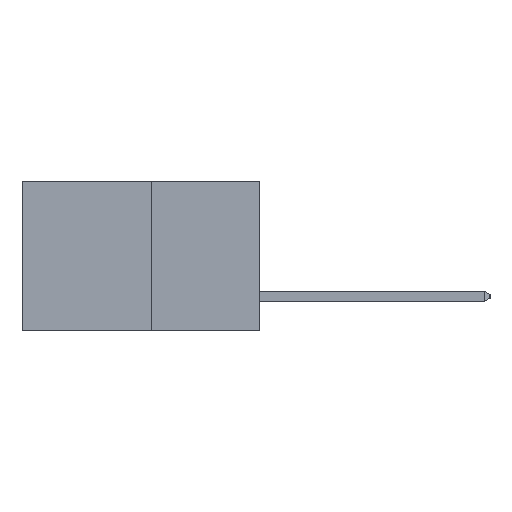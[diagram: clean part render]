
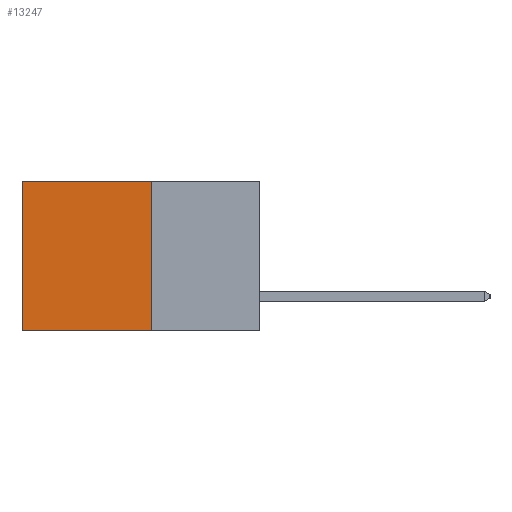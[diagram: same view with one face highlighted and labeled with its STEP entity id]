
A CAD part, left-side view. The second image highlights one B-rep face of the part: STEP entity #13247.
In plain terms, the highlighted planar face has unit normal (-1, 0, 0).
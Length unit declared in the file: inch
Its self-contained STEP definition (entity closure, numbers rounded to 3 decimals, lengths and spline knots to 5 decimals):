
#35 = VECTOR ( 'NONE', #3221, 39.37008 ) ;
#95 = CARTESIAN_POINT ( 'NONE',  ( 0.277, 0.27, -0.37 ) ) ;
#238 = ORIENTED_EDGE ( 'NONE', *, *, #1452, .F. ) ;
#782 = DIRECTION ( 'NONE',  ( 0., 1., 0. ) ) ;
#844 = CARTESIAN_POINT ( 'NONE',  ( 0.277, 0.59, -0.37 ) ) ;
#1452 = EDGE_CURVE ( 'NONE', #14737, #11930, #11901, .T. ) ;
#1801 = EDGE_CURVE ( 'NONE', #3575, #6230, #9563, .T. ) ;
#3221 = DIRECTION ( 'NONE',  ( 0., 0., -1. ) ) ;
#3575 = VERTEX_POINT ( 'NONE', #13054 ) ;
#3719 = FACE_OUTER_BOUND ( 'NONE', #7787, .T. ) ;
#3746 = PLANE ( 'NONE',  #14738 ) ;
#3775 = CARTESIAN_POINT ( 'NONE',  ( 0.277, 0.59, -0.37 ) ) ;
#4943 = DIRECTION ( 'NONE',  ( 1., 0., 0. ) ) ;
#5330 = CARTESIAN_POINT ( 'NONE',  ( 0.277, 0.27, -0.37 ) ) ;
#6230 = VERTEX_POINT ( 'NONE', #844 ) ;
#6769 = CARTESIAN_POINT ( 'NONE',  ( 0.277, 0.27, -0.37 ) ) ;
#6771 = ORIENTED_EDGE ( 'NONE', *, *, #14100, .F. ) ;
#6775 = CARTESIAN_POINT ( 'NONE',  ( 0.277, 0.27, 0. ) ) ;
#6854 = VECTOR ( 'NONE', #12312, 39.37008 ) ;
#7787 = EDGE_LOOP ( 'NONE', ( #9128, #6771, #238, #8136 ) ) ;
#7995 = CARTESIAN_POINT ( 'NONE',  ( 0.277, 0.27, 0. ) ) ;
#8136 = ORIENTED_EDGE ( 'NONE', *, *, #14145, .T. ) ;
#8541 = CARTESIAN_POINT ( 'NONE',  ( 0.277, 0.27, -0.37 ) ) ;
#9128 = ORIENTED_EDGE ( 'NONE', *, *, #1801, .T. ) ;
#9257 = LINE ( 'NONE', #7995, #12634 ) ;
#9506 = DIRECTION ( 'NONE',  ( 0., 0., -1. ) ) ;
#9563 = LINE ( 'NONE', #3775, #35 ) ;
#11172 = VECTOR ( 'NONE', #9506, 39.37008 ) ;
#11901 = LINE ( 'NONE', #6769, #11172 ) ;
#11930 = VERTEX_POINT ( 'NONE', #8541 ) ;
#12312 = DIRECTION ( 'NONE',  ( 0., 1., 0. ) ) ;
#12634 = VECTOR ( 'NONE', #782, 39.37008 ) ;
#13000 = LINE ( 'NONE', #5330, #6854 ) ;
#13054 = CARTESIAN_POINT ( 'NONE',  ( 0.277, 0.59, 0. ) ) ;
#13078 = DIRECTION ( 'NONE',  ( 0., 0., -1. ) ) ;
#13247 = ADVANCED_FACE ( 'NONE', ( #3719 ), #3746, .F. ) ;
#14100 = EDGE_CURVE ( 'NONE', #11930, #6230, #13000, .T. ) ;
#14145 = EDGE_CURVE ( 'NONE', #14737, #3575, #9257, .T. ) ;
#14737 = VERTEX_POINT ( 'NONE', #6775 ) ;
#14738 = AXIS2_PLACEMENT_3D ( 'NONE', #95, #4943, #13078 ) ;
